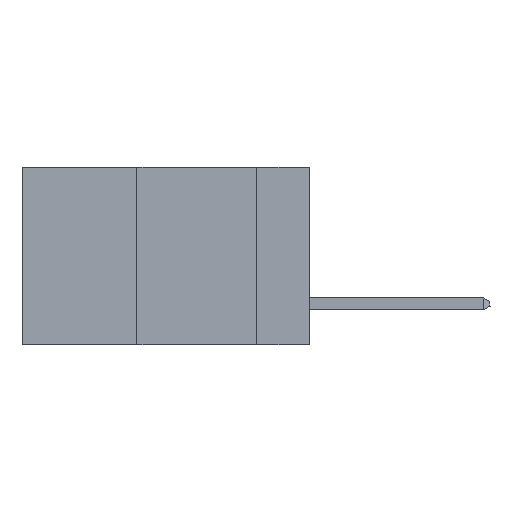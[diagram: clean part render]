
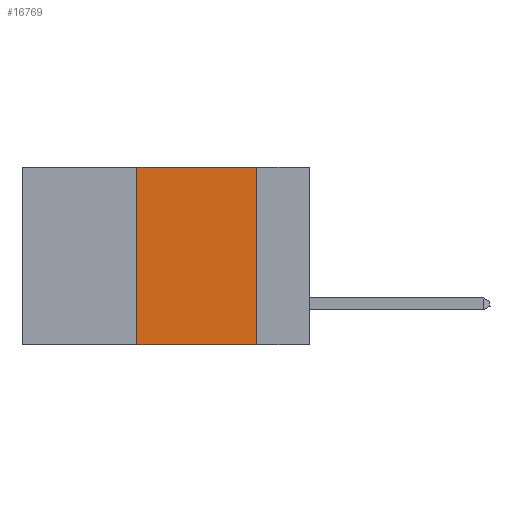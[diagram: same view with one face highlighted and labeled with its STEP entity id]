
A CAD part, left-side view. The second image highlights one B-rep face of the part: STEP entity #16769.
In plain terms, the highlighted planar face has unit normal (-1, 0, 0).
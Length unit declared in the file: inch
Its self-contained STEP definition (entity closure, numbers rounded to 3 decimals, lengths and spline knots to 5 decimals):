
#2975 = VERTEX_POINT ( 'NONE', #22171 ) ;
#3403 = CARTESIAN_POINT ( 'NONE',  ( 0., 0.11, -0.37 ) ) ;
#3979 = DIRECTION ( 'NONE',  ( 0., 0., -1. ) ) ;
#4415 = CARTESIAN_POINT ( 'NONE',  ( 0., 0.6, -0.37 ) ) ;
#5656 = CARTESIAN_POINT ( 'NONE',  ( 0., 0.6, 0. ) ) ;
#6685 = VERTEX_POINT ( 'NONE', #3403 ) ;
#7030 = VECTOR ( 'NONE', #20406, 39.37008 ) ;
#7144 = VERTEX_POINT ( 'NONE', #16986 ) ;
#8086 = ORIENTED_EDGE ( 'NONE', *, *, #13764, .F. ) ;
#8489 = DIRECTION ( 'NONE',  ( 0., -1., 0. ) ) ;
#10207 = VERTEX_POINT ( 'NONE', #21902 ) ;
#10274 = DIRECTION ( 'NONE',  ( 0., 0., -1. ) ) ;
#10536 = CARTESIAN_POINT ( 'NONE',  ( 0., 0.11, 0. ) ) ;
#11212 = ORIENTED_EDGE ( 'NONE', *, *, #24291, .T. ) ;
#11869 = PLANE ( 'NONE',  #18393 ) ;
#12516 = EDGE_CURVE ( 'NONE', #7144, #2975, #18336, .T. ) ;
#12976 = VECTOR ( 'NONE', #23323, 39.37008 ) ;
#13236 = LINE ( 'NONE', #10536, #23412 ) ;
#13611 = LINE ( 'NONE', #19181, #12976 ) ;
#13764 = EDGE_CURVE ( 'NONE', #2975, #6685, #13236, .T. ) ;
#13902 = DIRECTION ( 'NONE',  ( 1., 0., 0. ) ) ;
#14335 = VECTOR ( 'NONE', #8489, 39.37008 ) ;
#16769 = ADVANCED_FACE ( 'NONE', ( #18428 ), #11869, .F. ) ;
#16986 = CARTESIAN_POINT ( 'NONE',  ( 0., 0.36, 0. ) ) ;
#18336 = LINE ( 'NONE', #22804, #7030 ) ;
#18393 = AXIS2_PLACEMENT_3D ( 'NONE', #5656, #13902, #3979 ) ;
#18428 = FACE_OUTER_BOUND ( 'NONE', #18728, .T. ) ;
#18592 = EDGE_CURVE ( 'NONE', #10207, #7144, #13611, .T. ) ;
#18728 = EDGE_LOOP ( 'NONE', ( #8086, #20697, #21771, #11212 ) ) ;
#19181 = CARTESIAN_POINT ( 'NONE',  ( 0., 0.36, 0. ) ) ;
#20406 = DIRECTION ( 'NONE',  ( 0., -1., 0. ) ) ;
#20697 = ORIENTED_EDGE ( 'NONE', *, *, #12516, .F. ) ;
#20987 = LINE ( 'NONE', #4415, #14335 ) ;
#21771 = ORIENTED_EDGE ( 'NONE', *, *, #18592, .F. ) ;
#21902 = CARTESIAN_POINT ( 'NONE',  ( 0., 0.36, -0.37 ) ) ;
#22171 = CARTESIAN_POINT ( 'NONE',  ( 0., 0.11, 0. ) ) ;
#22804 = CARTESIAN_POINT ( 'NONE',  ( 0., 0.6, 0. ) ) ;
#23323 = DIRECTION ( 'NONE',  ( 0., 0., 1. ) ) ;
#23412 = VECTOR ( 'NONE', #10274, 39.37008 ) ;
#24291 = EDGE_CURVE ( 'NONE', #10207, #6685, #20987, .T. ) ;
